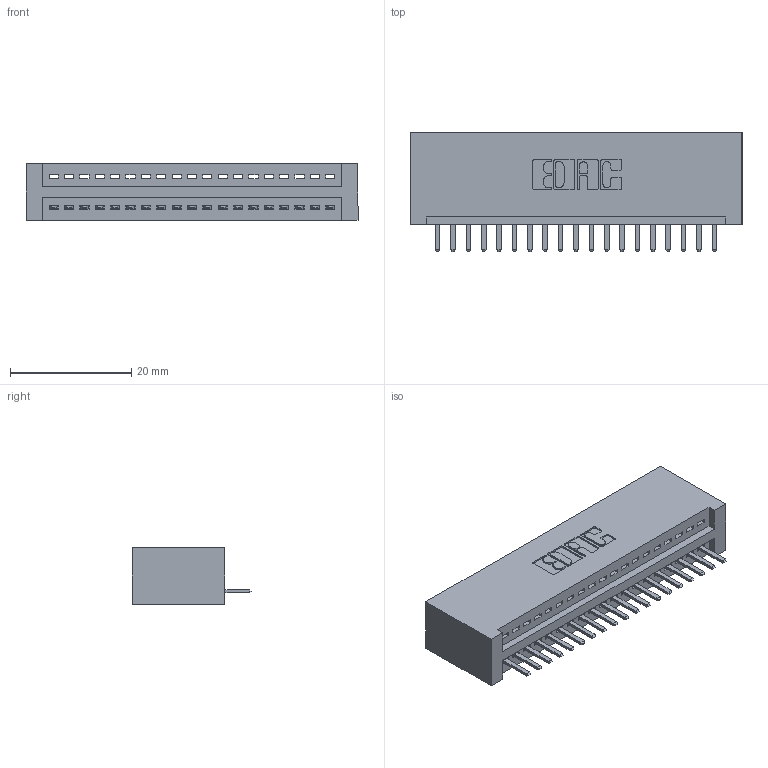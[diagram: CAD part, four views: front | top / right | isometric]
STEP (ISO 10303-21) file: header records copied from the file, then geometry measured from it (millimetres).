
FILE_DESCRIPTION (( 'STEP AP203' ), '1' );
FILE_NAME ('395-019-520-101.STEP', '2019-10-17T16:31:53', ( '' ), ( '' ), 'SwSTEP 2.0', 'SolidWorks 2016', '' );
FILE_SCHEMA (( 'CONFIG_CONTROL_DESIGN' ));
Length unit declared in the file: inch
Products named in the file (3): 395-019-520-101; 345-292-001_345-293-120; 345 Part_No Mounting Lugs
Assembly tree (20 placements, depth 2):
  395-019-520-101
    345 Part_No Mounting Lugs
    345-292-001_345-293-120  x19
Bounding box: 54.86 x 19.68 x 9.4 mm (x, y, z)
Volume: 5552.3 mm3; surface area: 7077.3 mm2
Topology: 20 solids, 20 shells, 1296 faces, 3813 edges, 2490 vertices
Faces by surface type: plane 874, cylinder 422
Entity records: 17233 total; most frequent: CARTESIAN_POINT 3005, ORIENTED_EDGE 2946, DIRECTION 2639, EDGE_CURVE 1473, LINE 1269, VECTOR 1269, VERTEX_POINT 978, AXIS2_PLACEMENT_3D 685
